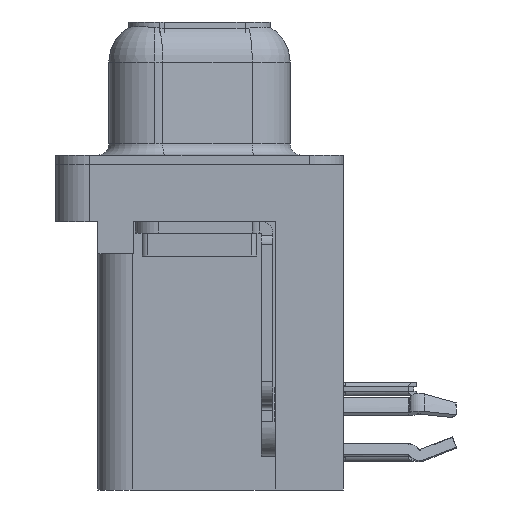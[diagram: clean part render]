
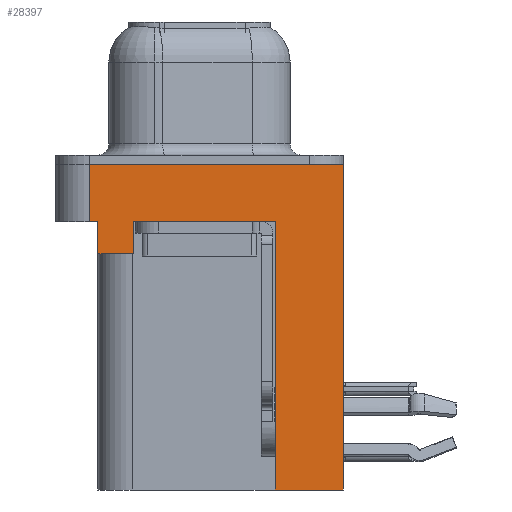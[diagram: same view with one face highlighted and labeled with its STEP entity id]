
A CAD part, left-side view. The second image highlights one B-rep face of the part: STEP entity #28397.
In plain terms, the highlighted planar face has unit normal (-1, 0, 0).
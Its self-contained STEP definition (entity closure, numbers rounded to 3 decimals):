
#340 = DIRECTION ( 'NONE',  ( 0., 1., 0. ) ) ;
#1763 = VERTEX_POINT ( 'NONE', #29280 ) ;
#1945 = EDGE_CURVE ( 'NONE', #22331, #33859, #18896, .T. ) ;
#2696 = LINE ( 'NONE', #22764, #9584 ) ;
#3877 = VERTEX_POINT ( 'NONE', #9645 ) ;
#4369 = EDGE_CURVE ( 'NONE', #10643, #6648, #8916, .T. ) ;
#4460 = VERTEX_POINT ( 'NONE', #24407 ) ;
#5409 = EDGE_LOOP ( 'NONE', ( #17717, #35998, #26950, #31782, #23280, #19482, #8941, #6766, #36134, #34112 ) ) ;
#6648 = VERTEX_POINT ( 'NONE', #6917 ) ;
#6766 = ORIENTED_EDGE ( 'NONE', *, *, #15489, .F. ) ;
#6917 = CARTESIAN_POINT ( 'NONE',  ( -2.91, -3.295, -2.5 ) ) ;
#7592 = DIRECTION ( 'NONE',  ( 0., 0., 1. ) ) ;
#8056 = VECTOR ( 'NONE', #36652, 1000. ) ;
#8285 = EDGE_CURVE ( 'NONE', #14588, #3877, #8308, .T. ) ;
#8308 = LINE ( 'NONE', #16752, #12181 ) ;
#8916 = LINE ( 'NONE', #34360, #10244 ) ;
#8941 = ORIENTED_EDGE ( 'NONE', *, *, #4369, .T. ) ;
#9398 = VECTOR ( 'NONE', #7592, 1000. ) ;
#9584 = VECTOR ( 'NONE', #37664, 1000. ) ;
#9645 = CARTESIAN_POINT ( 'NONE',  ( -2.91, -6.275, 0. ) ) ;
#10244 = VECTOR ( 'NONE', #22887, 1000. ) ;
#10643 = VERTEX_POINT ( 'NONE', #35077 ) ;
#10714 = DIRECTION ( 'NONE',  ( 0., 0., 1. ) ) ;
#12181 = VECTOR ( 'NONE', #27834, 1000. ) ;
#12352 = AXIS2_PLACEMENT_3D ( 'NONE', #28112, #13584, #10714 ) ;
#12519 = LINE ( 'NONE', #18269, #13275 ) ;
#13141 = LINE ( 'NONE', #36086, #14094 ) ;
#13275 = VECTOR ( 'NONE', #27231, 1000. ) ;
#13367 = DIRECTION ( 'NONE',  ( 0., 0., 1. ) ) ;
#13584 = DIRECTION ( 'NONE',  ( -1., 0., 0. ) ) ;
#14094 = VECTOR ( 'NONE', #18702, 1000. ) ;
#14588 = VERTEX_POINT ( 'NONE', #33237 ) ;
#15241 = CARTESIAN_POINT ( 'NONE',  ( -2.91, -3.295, -14.2 ) ) ;
#15489 = EDGE_CURVE ( 'NONE', #4460, #6648, #37233, .T. ) ;
#15491 = CARTESIAN_POINT ( 'NONE',  ( -2.91, 4.775, -2.5 ) ) ;
#16251 = CARTESIAN_POINT ( 'NONE',  ( -2.91, 4.425, -3.9 ) ) ;
#16464 = PLANE ( 'NONE',  #12352 ) ;
#16591 = CARTESIAN_POINT ( 'NONE',  ( -2.91, 4.775, -2.5 ) ) ;
#16752 = CARTESIAN_POINT ( 'NONE',  ( -2.91, -6.275, -2.5 ) ) ;
#16753 = EDGE_CURVE ( 'NONE', #14588, #4460, #33007, .T. ) ;
#17717 = ORIENTED_EDGE ( 'NONE', *, *, #22269, .F. ) ;
#18269 = CARTESIAN_POINT ( 'NONE',  ( -2.91, 4.425, -3.9 ) ) ;
#18702 = DIRECTION ( 'NONE',  ( 0., -1., 0. ) ) ;
#18896 = LINE ( 'NONE', #16591, #9398 ) ;
#19482 = ORIENTED_EDGE ( 'NONE', *, *, #29797, .T. ) ;
#21400 = EDGE_CURVE ( 'NONE', #27349, #1763, #12519, .T. ) ;
#22269 = EDGE_CURVE ( 'NONE', #33859, #3877, #2696, .T. ) ;
#22331 = VERTEX_POINT ( 'NONE', #15491 ) ;
#22696 = CARTESIAN_POINT ( 'NONE',  ( -2.91, -3.295, -14.2 ) ) ;
#22764 = CARTESIAN_POINT ( 'NONE',  ( -2.91, -6.275, 0. ) ) ;
#22887 = DIRECTION ( 'NONE',  ( 0., -1., 0. ) ) ;
#23280 = ORIENTED_EDGE ( 'NONE', *, *, #21400, .F. ) ;
#24407 = CARTESIAN_POINT ( 'NONE',  ( -2.91, -3.295, -14.2 ) ) ;
#24623 = LINE ( 'NONE', #31108, #8056 ) ;
#25045 = FACE_OUTER_BOUND ( 'NONE', #5409, .T. ) ;
#25368 = VERTEX_POINT ( 'NONE', #29908 ) ;
#26950 = ORIENTED_EDGE ( 'NONE', *, *, #37277, .T. ) ;
#27231 = DIRECTION ( 'NONE',  ( 0., 1., 0. ) ) ;
#27349 = VERTEX_POINT ( 'NONE', #31532 ) ;
#27834 = DIRECTION ( 'NONE',  ( 0., 0., 1. ) ) ;
#28112 = CARTESIAN_POINT ( 'NONE',  ( -2.91, -6.275, -2.5 ) ) ;
#28397 = ADVANCED_FACE ( 'NONE', ( #25045 ), #16464, .T. ) ;
#29280 = CARTESIAN_POINT ( 'NONE',  ( -2.91, 4.425, -3.9 ) ) ;
#29797 = EDGE_CURVE ( 'NONE', #27349, #10643, #24623, .T. ) ;
#29908 = CARTESIAN_POINT ( 'NONE',  ( -2.91, 4.425, -2.5 ) ) ;
#31108 = CARTESIAN_POINT ( 'NONE',  ( -2.91, 2.895, -3.9 ) ) ;
#31532 = CARTESIAN_POINT ( 'NONE',  ( -2.91, 2.895, -3.9 ) ) ;
#31782 = ORIENTED_EDGE ( 'NONE', *, *, #36986, .F. ) ;
#32333 = CARTESIAN_POINT ( 'NONE',  ( -2.91, 4.775, 0. ) ) ;
#33007 = LINE ( 'NONE', #15241, #35708 ) ;
#33237 = CARTESIAN_POINT ( 'NONE',  ( -2.91, -6.275, -14.2 ) ) ;
#33260 = LINE ( 'NONE', #16251, #34854 ) ;
#33859 = VERTEX_POINT ( 'NONE', #32333 ) ;
#34112 = ORIENTED_EDGE ( 'NONE', *, *, #8285, .T. ) ;
#34359 = DIRECTION ( 'NONE',  ( 0., 0., 1. ) ) ;
#34360 = CARTESIAN_POINT ( 'NONE',  ( -2.91, -6.275, -2.5 ) ) ;
#34854 = VECTOR ( 'NONE', #13367, 1000. ) ;
#35077 = CARTESIAN_POINT ( 'NONE',  ( -2.91, 2.895, -2.5 ) ) ;
#35661 = VECTOR ( 'NONE', #34359, 1000. ) ;
#35708 = VECTOR ( 'NONE', #340, 1000. ) ;
#35998 = ORIENTED_EDGE ( 'NONE', *, *, #1945, .F. ) ;
#36086 = CARTESIAN_POINT ( 'NONE',  ( -2.91, -6.275, -2.5 ) ) ;
#36134 = ORIENTED_EDGE ( 'NONE', *, *, #16753, .F. ) ;
#36652 = DIRECTION ( 'NONE',  ( 0., 0., 1. ) ) ;
#36986 = EDGE_CURVE ( 'NONE', #1763, #25368, #33260, .T. ) ;
#37233 = LINE ( 'NONE', #22696, #35661 ) ;
#37277 = EDGE_CURVE ( 'NONE', #22331, #25368, #13141, .T. ) ;
#37664 = DIRECTION ( 'NONE',  ( 0., -1., 0. ) ) ;
